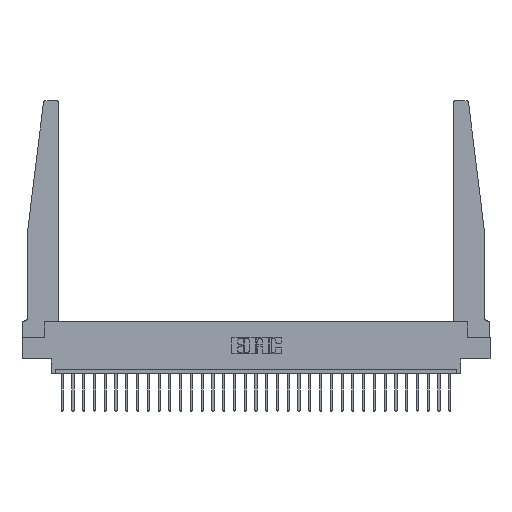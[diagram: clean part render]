
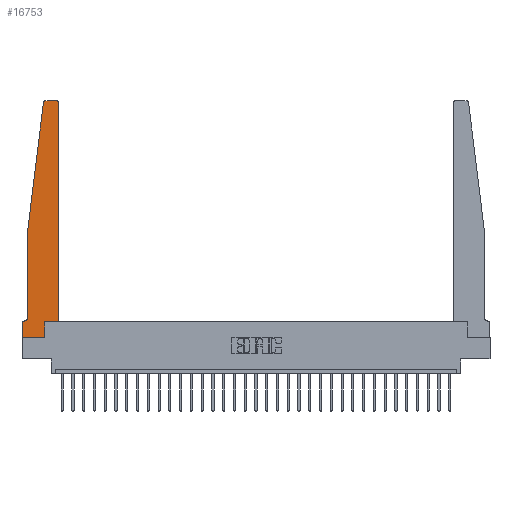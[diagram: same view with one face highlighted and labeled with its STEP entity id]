
A CAD part, top view. The second image highlights one B-rep face of the part: STEP entity #16753.
In plain terms, the highlighted planar face has unit normal (0, 0, 1).
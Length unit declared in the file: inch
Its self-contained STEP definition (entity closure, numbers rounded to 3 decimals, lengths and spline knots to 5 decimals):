
#397 = EDGE_CURVE ( 'NONE', #28030, #16967, #11651, .T. ) ;
#904 = DIRECTION ( 'NONE',  ( 0., -1., 0. ) ) ;
#1210 = DIRECTION ( 'NONE',  ( -1., 0., 0. ) ) ;
#2173 = VECTOR ( 'NONE', #7784, 39.37008 ) ;
#2400 = VERTEX_POINT ( 'NONE', #21881 ) ;
#2495 = CARTESIAN_POINT ( 'NONE',  ( 0.2605, 0., 0.37 ) ) ;
#2672 = EDGE_CURVE ( 'NONE', #14004, #2400, #25826, .T. ) ;
#2943 = EDGE_LOOP ( 'NONE', ( #13117, #4734, #20972, #21597, #12418, #21991, #27802, #20667, #8636, #15203, #23395, #15826 ) ) ;
#2958 = CARTESIAN_POINT ( 'NONE',  ( 0., 0.1875, 0.37 ) ) ;
#3525 = DIRECTION ( 'NONE',  ( 1., 0., 0. ) ) ;
#4172 = AXIS2_PLACEMENT_3D ( 'NONE', #13491, #13790, #27373 ) ;
#4551 = CARTESIAN_POINT ( 'NONE',  ( 0.27653, 2.72, 0.37 ) ) ;
#4672 = DIRECTION ( 'NONE',  ( 0., 0., 1. ) ) ;
#4734 = ORIENTED_EDGE ( 'NONE', *, *, #22852, .T. ) ;
#4814 = CARTESIAN_POINT ( 'NONE',  ( 0.065, 1.25, 0.37 ) ) ;
#5542 = EDGE_CURVE ( 'NONE', #2400, #28030, #8897, .T. ) ;
#5867 = EDGE_CURVE ( 'NONE', #16967, #8173, #7942, .T. ) ;
#6875 = PLANE ( 'NONE',  #17907 ) ;
#6903 = DIRECTION ( 'NONE',  ( 1., 0., 0. ) ) ;
#6984 = VECTOR ( 'NONE', #18149, 39.37008 ) ;
#7099 = CARTESIAN_POINT ( 'NONE',  ( 0.015, 0.2375, 0.37 ) ) ;
#7770 = CARTESIAN_POINT ( 'NONE',  ( 0.065, 0.2375, 0.37 ) ) ;
#7784 = DIRECTION ( 'NONE',  ( -1., 0., 0. ) ) ;
#7942 = CIRCLE ( 'NONE', #4172, 0.03 ) ;
#8173 = VERTEX_POINT ( 'NONE', #28273 ) ;
#8333 = EDGE_CURVE ( 'NONE', #22459, #10979, #28643, .T. ) ;
#8510 = EDGE_CURVE ( 'NONE', #8173, #16867, #27188, .T. ) ;
#8538 = CARTESIAN_POINT ( 'NONE',  ( 0.065, 1.25, 0.37 ) ) ;
#8570 = EDGE_CURVE ( 'NONE', #10979, #24923, #16884, .T. ) ;
#8636 = ORIENTED_EDGE ( 'NONE', *, *, #2672, .T. ) ;
#8897 = LINE ( 'NONE', #22977, #6984 ) ;
#9163 = VECTOR ( 'NONE', #11368, 39.37008 ) ;
#9587 = CARTESIAN_POINT ( 'NONE',  ( 0.425, 2.72, 0.37 ) ) ;
#9657 = DIRECTION ( 'NONE',  ( 0., -1., 0. ) ) ;
#9976 = VECTOR ( 'NONE', #1210, 39.37008 ) ;
#10365 = CARTESIAN_POINT ( 'NONE',  ( 0.2605, 0.18, 0.37 ) ) ;
#10414 = LINE ( 'NONE', #28370, #21475 ) ;
#10566 = EDGE_CURVE ( 'NONE', #22535, #14004, #10414, .T. ) ;
#10979 = VERTEX_POINT ( 'NONE', #4814 ) ;
#11368 = DIRECTION ( 'NONE',  ( 0., 1., 0. ) ) ;
#11651 = LINE ( 'NONE', #15806, #9163 ) ;
#11983 = EDGE_CURVE ( 'NONE', #24923, #22158, #26466, .T. ) ;
#12418 = ORIENTED_EDGE ( 'NONE', *, *, #11983, .T. ) ;
#13117 = ORIENTED_EDGE ( 'NONE', *, *, #8510, .T. ) ;
#13491 = CARTESIAN_POINT ( 'NONE',  ( 0.395, 2.72, 0.37 ) ) ;
#13790 = DIRECTION ( 'NONE',  ( 0., 0., 1. ) ) ;
#14004 = VERTEX_POINT ( 'NONE', #2495 ) ;
#14654 = CARTESIAN_POINT ( 'NONE',  ( 0.065, 1.25, 0.37 ) ) ;
#15203 = ORIENTED_EDGE ( 'NONE', *, *, #5542, .T. ) ;
#15642 = CARTESIAN_POINT ( 'NONE',  ( 0.27653, 2.75, 0.37 ) ) ;
#15806 = CARTESIAN_POINT ( 'NONE',  ( 0.425, 0.18, 0.37 ) ) ;
#15826 = ORIENTED_EDGE ( 'NONE', *, *, #5867, .T. ) ;
#16640 = CARTESIAN_POINT ( 'NONE',  ( 0.24675, 2.72367, 0.37 ) ) ;
#16753 = ADVANCED_FACE ( 'NONE', ( #26996 ), #6875, .T. ) ;
#16867 = VERTEX_POINT ( 'NONE', #15642 ) ;
#16884 = LINE ( 'NONE', #14654, #18142 ) ;
#16967 = VERTEX_POINT ( 'NONE', #9587 ) ;
#17661 = DIRECTION ( 'NONE',  ( -1., 0., 0. ) ) ;
#17907 = AXIS2_PLACEMENT_3D ( 'NONE', #24779, #4672, #22589 ) ;
#18142 = VECTOR ( 'NONE', #9657, 39.37008 ) ;
#18149 = DIRECTION ( 'NONE',  ( 1., 0., 0. ) ) ;
#18883 = EDGE_CURVE ( 'NONE', #22158, #21634, #19007, .T. ) ;
#18946 = VECTOR ( 'NONE', #904, 39.37008 ) ;
#18977 = AXIS2_PLACEMENT_3D ( 'NONE', #7099, #22215, #17661 ) ;
#19007 = LINE ( 'NONE', #19285, #9976 ) ;
#19173 = EDGE_CURVE ( 'NONE', #21634, #22535, #20901, .T. ) ;
#19285 = CARTESIAN_POINT ( 'NONE',  ( 0.065, 0.1875, 0.37 ) ) ;
#20184 = CARTESIAN_POINT ( 'NONE',  ( 0., 0., 0.37 ) ) ;
#20218 = AXIS2_PLACEMENT_3D ( 'NONE', #4551, #22472, #6903 ) ;
#20667 = ORIENTED_EDGE ( 'NONE', *, *, #10566, .T. ) ;
#20901 = LINE ( 'NONE', #25287, #18946 ) ;
#20972 = ORIENTED_EDGE ( 'NONE', *, *, #8333, .T. ) ;
#21252 = CARTESIAN_POINT ( 'NONE',  ( 0.015, 0.1875, 0.37 ) ) ;
#21475 = VECTOR ( 'NONE', #3525, 39.37008 ) ;
#21597 = ORIENTED_EDGE ( 'NONE', *, *, #8570, .T. ) ;
#21634 = VERTEX_POINT ( 'NONE', #2958 ) ;
#21881 = CARTESIAN_POINT ( 'NONE',  ( 0.2605, 0.18, 0.37 ) ) ;
#21884 = VECTOR ( 'NONE', #24255, 39.37008 ) ;
#21991 = ORIENTED_EDGE ( 'NONE', *, *, #18883, .T. ) ;
#22158 = VERTEX_POINT ( 'NONE', #21252 ) ;
#22215 = DIRECTION ( 'NONE',  ( 0., 0., -1. ) ) ;
#22459 = VERTEX_POINT ( 'NONE', #16640 ) ;
#22472 = DIRECTION ( 'NONE',  ( 0., 0., 1. ) ) ;
#22535 = VERTEX_POINT ( 'NONE', #20184 ) ;
#22589 = DIRECTION ( 'NONE',  ( 1., 0., 0. ) ) ;
#22852 = EDGE_CURVE ( 'NONE', #16867, #22459, #28626, .T. ) ;
#22977 = CARTESIAN_POINT ( 'NONE',  ( 0.425, 0.18, 0.37 ) ) ;
#23328 = CARTESIAN_POINT ( 'NONE',  ( 0.25, 2.75, 0.37 ) ) ;
#23395 = ORIENTED_EDGE ( 'NONE', *, *, #397, .T. ) ;
#24255 = DIRECTION ( 'NONE',  ( -0.122, -0.992, 0. ) ) ;
#24779 = CARTESIAN_POINT ( 'NONE',  ( 0., 0.1875, 0.37 ) ) ;
#24923 = VERTEX_POINT ( 'NONE', #7770 ) ;
#25287 = CARTESIAN_POINT ( 'NONE',  ( 0., 0., 0.37 ) ) ;
#25826 = LINE ( 'NONE', #10365, #28615 ) ;
#26466 = CIRCLE ( 'NONE', #18977, 0.05 ) ;
#26996 = FACE_OUTER_BOUND ( 'NONE', #2943, .T. ) ;
#27188 = LINE ( 'NONE', #23328, #2173 ) ;
#27373 = DIRECTION ( 'NONE',  ( 1., 0., 0. ) ) ;
#27802 = ORIENTED_EDGE ( 'NONE', *, *, #19173, .T. ) ;
#28019 = CARTESIAN_POINT ( 'NONE',  ( 0.425, 0.18, 0.37 ) ) ;
#28030 = VERTEX_POINT ( 'NONE', #28019 ) ;
#28273 = CARTESIAN_POINT ( 'NONE',  ( 0.395, 2.75, 0.37 ) ) ;
#28318 = DIRECTION ( 'NONE',  ( 0., 1., 0. ) ) ;
#28370 = CARTESIAN_POINT ( 'NONE',  ( 0., 0., 0.37 ) ) ;
#28615 = VECTOR ( 'NONE', #28318, 39.37008 ) ;
#28626 = CIRCLE ( 'NONE', #20218, 0.03 ) ;
#28643 = LINE ( 'NONE', #8538, #21884 ) ;
